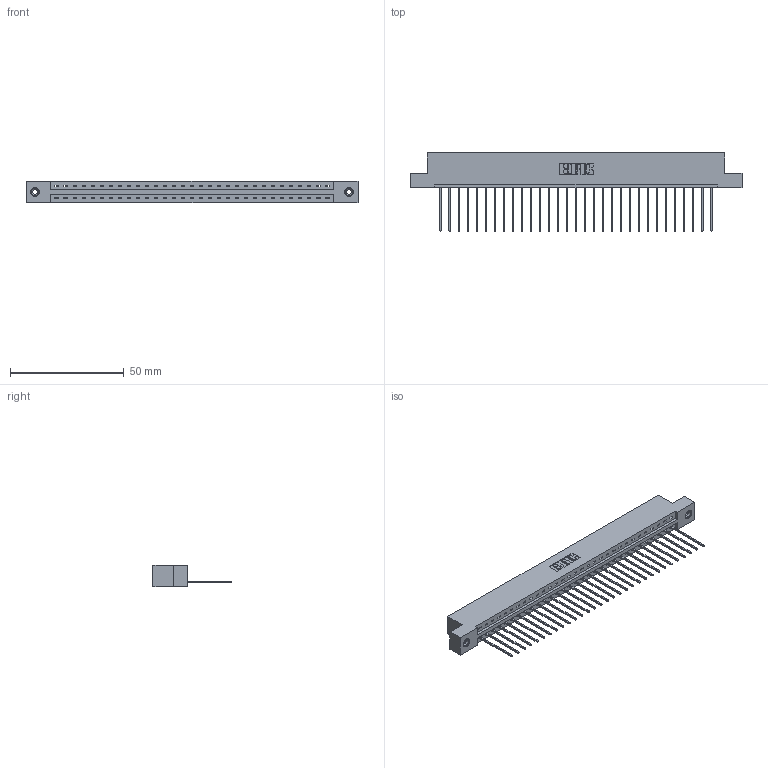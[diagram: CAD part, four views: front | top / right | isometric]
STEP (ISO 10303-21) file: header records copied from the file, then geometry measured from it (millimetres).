
FILE_DESCRIPTION (( 'STEP AP203' ), '1' );
FILE_NAME ('337-031-541-108.STEP', '2018-08-07T03:33:25', ( '' ), ( '' ), 'SwSTEP 2.0', 'SolidWorks 2016', '' );
FILE_SCHEMA (( 'CONFIG_CONTROL_DESIGN' ));
Length unit declared in the file: inch
Products named in the file (4): 337 Part_Flush Mounting Lugs - 0.156 Dia-TI; 345-292-001_345-293-141; 345-250-001_345-250-003-102; 337-031-541-108
Assembly tree (34 placements, depth 2):
  337-031-541-108
    337 Part_Flush Mounting Lugs - 0.156 Dia-TI
    345-292-001_345-293-141  x31
    345-250-001_345-250-003-102  x2
Bounding box: 145.85 x 34.3 x 9.4 mm (x, y, z)
Volume: 15116.5 mm3; surface area: 16218.5 mm2
Topology: 34 solids, 34 shells, 2096 faces, 6275 edges, 4134 vertices
Faces by surface type: plane 1528, cylinder 552, cone 12, torus 4
Entity records: 25670 total; most frequent: CARTESIAN_POINT 4450, ORIENTED_EDGE 4410, DIRECTION 3801, EDGE_CURVE 2205, VECTOR 2057, LINE 2057, VERTEX_POINT 1464, AXIS2_PLACEMENT_3D 872
